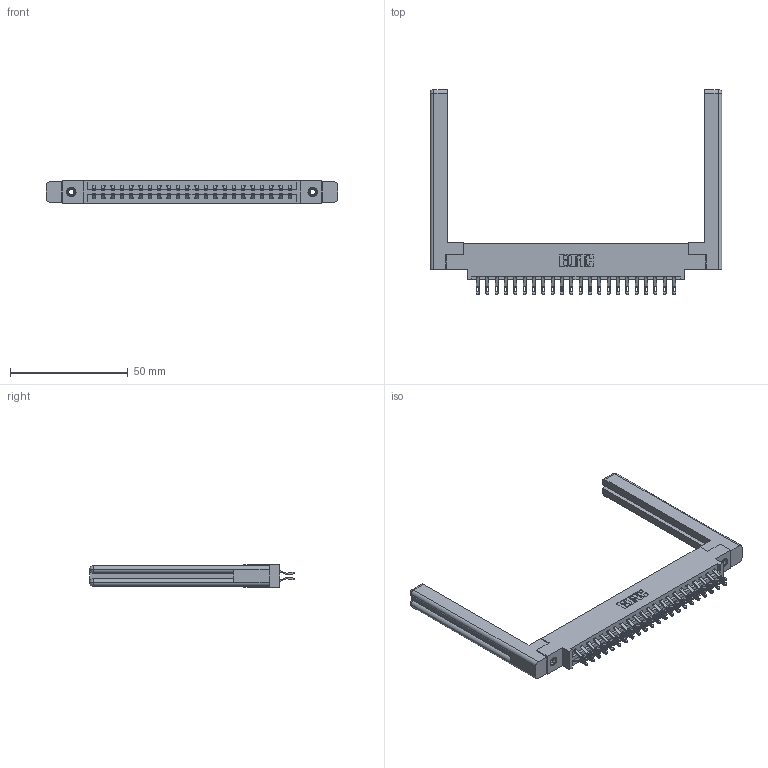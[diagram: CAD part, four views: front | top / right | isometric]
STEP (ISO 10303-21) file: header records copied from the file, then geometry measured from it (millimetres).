
FILE_DESCRIPTION (( 'STEP AP203' ), '1' );
FILE_NAME ('387-044-555-858.STEP', '2019-10-18T06:15:34', ( '' ), ( '' ), 'SwSTEP 2.0', 'SolidWorks 2016', '' );
FILE_SCHEMA (( 'CONFIG_CONTROL_DESIGN' ));
Length unit declared in the file: inch
Products named in the file (5): 345-292-001_555 Tail; 345-250-001_345-250-001-102; 387-044-555-858; 337 Part_0.170 Offset - 0.156 Dia-TI; 307-220-058
Assembly tree (49 placements, depth 2):
  387-044-555-858
    337 Part_0.170 Offset - 0.156 Dia-TI
    345-292-001_555 Tail  x44
    345-250-001_345-250-001-102  x2
    307-220-058  x2
Bounding box: 123.8 x 86.87 x 9.4 mm (x, y, z)
Volume: 19933.2 mm3; surface area: 19901.4 mm2
Topology: 49 solids, 49 shells, 2900 faces, 8993 edges, 5982 vertices
Faces by surface type: plane 1742, cylinder 1134, cone 12, torus 12
Entity records: 22736 total; most frequent: CARTESIAN_POINT 3891, ORIENTED_EDGE 3736, DIRECTION 3332, EDGE_CURVE 1868, VECTOR 1672, LINE 1672, VERTEX_POINT 1238, AXIS2_PLACEMENT_3D 830
